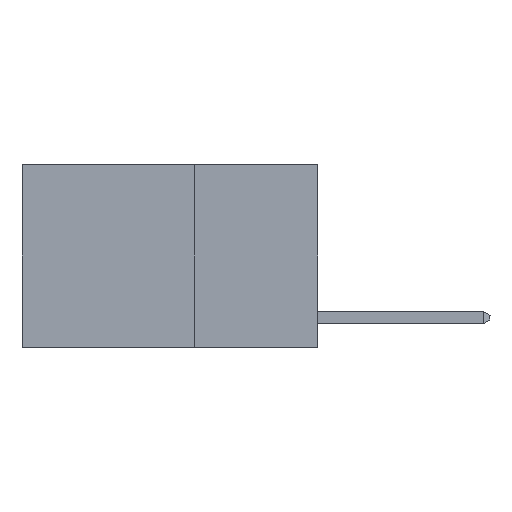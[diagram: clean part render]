
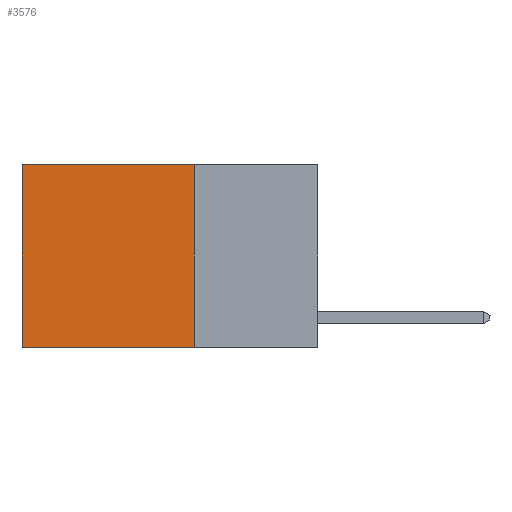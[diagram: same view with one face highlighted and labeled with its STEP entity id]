
A CAD part, left-side view. The second image highlights one B-rep face of the part: STEP entity #3576.
In plain terms, the highlighted planar face has unit normal (-1, 0, 0).
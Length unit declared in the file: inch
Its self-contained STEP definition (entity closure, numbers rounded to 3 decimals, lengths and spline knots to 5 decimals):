
#353 = DIRECTION ( 'NONE',  ( 0., 0., -1. ) ) ;
#412 = VERTEX_POINT ( 'NONE', #1017 ) ;
#450 = DIRECTION ( 'NONE',  ( 1., 0., 0. ) ) ;
#564 = PLANE ( 'NONE',  #3829 ) ;
#852 = CARTESIAN_POINT ( 'NONE',  ( 0.2625, 0.25, 0. ) ) ;
#1017 = CARTESIAN_POINT ( 'NONE',  ( 0.2625, 0.6, 0. ) ) ;
#1022 = CARTESIAN_POINT ( 'NONE',  ( 0.2625, 0.25, 0. ) ) ;
#1024 = CARTESIAN_POINT ( 'NONE',  ( 0.2625, 0.25, -0.37 ) ) ;
#1887 = LINE ( 'NONE', #9523, #15226 ) ;
#1999 = EDGE_CURVE ( 'NONE', #7166, #412, #3685, .T. ) ;
#2686 = EDGE_LOOP ( 'NONE', ( #12934, #4579, #5876, #7826 ) ) ;
#2979 = FACE_OUTER_BOUND ( 'NONE', #2686, .T. ) ;
#3576 = ADVANCED_FACE ( 'NONE', ( #2979 ), #564, .F. ) ;
#3685 = LINE ( 'NONE', #13574, #9964 ) ;
#3829 = AXIS2_PLACEMENT_3D ( 'NONE', #852, #450, #353 ) ;
#4579 = ORIENTED_EDGE ( 'NONE', *, *, #14024, .F. ) ;
#4597 = CARTESIAN_POINT ( 'NONE',  ( 0.2625, 0.6, -0.37 ) ) ;
#5153 = VERTEX_POINT ( 'NONE', #4597 ) ;
#5876 = ORIENTED_EDGE ( 'NONE', *, *, #11325, .F. ) ;
#7113 = VECTOR ( 'NONE', #10128, 39.37008 ) ;
#7166 = VERTEX_POINT ( 'NONE', #1022 ) ;
#7734 = DIRECTION ( 'NONE',  ( 0., 0., -1. ) ) ;
#7826 = ORIENTED_EDGE ( 'NONE', *, *, #1999, .T. ) ;
#7957 = LINE ( 'NONE', #16712, #7113 ) ;
#9523 = CARTESIAN_POINT ( 'NONE',  ( 0.2625, 0.25, -0.37 ) ) ;
#9964 = VECTOR ( 'NONE', #10466, 39.37008 ) ;
#10128 = DIRECTION ( 'NONE',  ( 0., 0., -1. ) ) ;
#10305 = LINE ( 'NONE', #15632, #14200 ) ;
#10466 = DIRECTION ( 'NONE',  ( 0., 1., 0. ) ) ;
#11325 = EDGE_CURVE ( 'NONE', #7166, #12041, #7957, .T. ) ;
#12041 = VERTEX_POINT ( 'NONE', #1024 ) ;
#12934 = ORIENTED_EDGE ( 'NONE', *, *, #13886, .T. ) ;
#13574 = CARTESIAN_POINT ( 'NONE',  ( 0.2625, 0.25, 0. ) ) ;
#13886 = EDGE_CURVE ( 'NONE', #412, #5153, #10305, .T. ) ;
#14024 = EDGE_CURVE ( 'NONE', #12041, #5153, #1887, .T. ) ;
#14200 = VECTOR ( 'NONE', #7734, 39.37008 ) ;
#14521 = DIRECTION ( 'NONE',  ( 0., 1., 0. ) ) ;
#15226 = VECTOR ( 'NONE', #14521, 39.37008 ) ;
#15632 = CARTESIAN_POINT ( 'NONE',  ( 0.2625, 0.6, 0. ) ) ;
#16712 = CARTESIAN_POINT ( 'NONE',  ( 0.2625, 0.25, 0. ) ) ;
